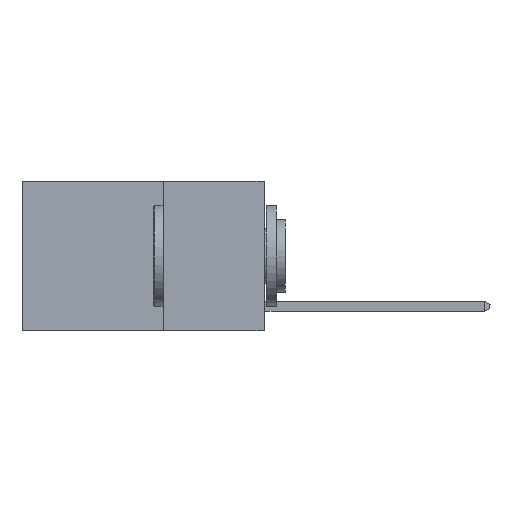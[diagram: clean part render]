
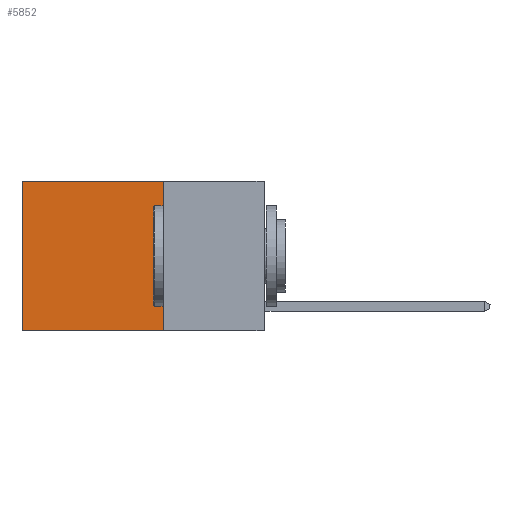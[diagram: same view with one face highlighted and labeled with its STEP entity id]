
A CAD part, left-side view. The second image highlights one B-rep face of the part: STEP entity #5852.
In plain terms, the highlighted planar face has unit normal (-1, 0, 0).
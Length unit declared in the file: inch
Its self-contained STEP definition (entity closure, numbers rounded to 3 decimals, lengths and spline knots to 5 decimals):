
#194 = DIRECTION ( 'NONE',  ( 0., 0., -1. ) ) ;
#208 = LINE ( 'NONE', #600, #21591 ) ;
#515 = EDGE_CURVE ( 'NONE', #6571, #20904, #5166, .T. ) ;
#600 = CARTESIAN_POINT ( 'NONE',  ( 0.2625, 0.25, 0. ) ) ;
#1303 = ORIENTED_EDGE ( 'NONE', *, *, #515, .T. ) ;
#1671 = EDGE_CURVE ( 'NONE', #5313, #13258, #208, .T. ) ;
#1845 = CARTESIAN_POINT ( 'NONE',  ( 0.2625, 0.25, -0.37 ) ) ;
#2308 = CARTESIAN_POINT ( 'NONE',  ( 0.2625, 0.6, 0. ) ) ;
#4271 = CARTESIAN_POINT ( 'NONE',  ( 0.2625, 0.25, -0.37 ) ) ;
#5166 = LINE ( 'NONE', #16009, #20101 ) ;
#5313 = VERTEX_POINT ( 'NONE', #15017 ) ;
#5852 = ADVANCED_FACE ( 'NONE', ( #8961 ), #7162, .F. ) ;
#6571 = VERTEX_POINT ( 'NONE', #2308 ) ;
#6863 = ORIENTED_EDGE ( 'NONE', *, *, #1671, .F. ) ;
#7162 = PLANE ( 'NONE',  #14867 ) ;
#8961 = FACE_OUTER_BOUND ( 'NONE', #11653, .T. ) ;
#9055 = CARTESIAN_POINT ( 'NONE',  ( 0.2625, 0.25, 0. ) ) ;
#9134 = DIRECTION ( 'NONE',  ( 1., 0., 0. ) ) ;
#9594 = EDGE_CURVE ( 'NONE', #13258, #20904, #16053, .T. ) ;
#11147 = DIRECTION ( 'NONE',  ( 0., 1., 0. ) ) ;
#11150 = ORIENTED_EDGE ( 'NONE', *, *, #14524, .T. ) ;
#11653 = EDGE_LOOP ( 'NONE', ( #1303, #23923, #6863, #11150 ) ) ;
#11856 = LINE ( 'NONE', #24598, #18808 ) ;
#13258 = VERTEX_POINT ( 'NONE', #1845 ) ;
#14524 = EDGE_CURVE ( 'NONE', #5313, #6571, #11856, .T. ) ;
#14867 = AXIS2_PLACEMENT_3D ( 'NONE', #9055, #9134, #24712 ) ;
#15017 = CARTESIAN_POINT ( 'NONE',  ( 0.2625, 0.25, 0. ) ) ;
#16009 = CARTESIAN_POINT ( 'NONE',  ( 0.2625, 0.6, 0. ) ) ;
#16053 = LINE ( 'NONE', #4271, #23964 ) ;
#16233 = DIRECTION ( 'NONE',  ( 0., 0., -1. ) ) ;
#18808 = VECTOR ( 'NONE', #11147, 39.37008 ) ;
#20101 = VECTOR ( 'NONE', #194, 39.37008 ) ;
#20215 = DIRECTION ( 'NONE',  ( 0., 1., 0. ) ) ;
#20904 = VERTEX_POINT ( 'NONE', #22861 ) ;
#21591 = VECTOR ( 'NONE', #16233, 39.37008 ) ;
#22861 = CARTESIAN_POINT ( 'NONE',  ( 0.2625, 0.6, -0.37 ) ) ;
#23923 = ORIENTED_EDGE ( 'NONE', *, *, #9594, .F. ) ;
#23964 = VECTOR ( 'NONE', #20215, 39.37008 ) ;
#24598 = CARTESIAN_POINT ( 'NONE',  ( 0.2625, 0.25, 0. ) ) ;
#24712 = DIRECTION ( 'NONE',  ( 0., 0., -1. ) ) ;
